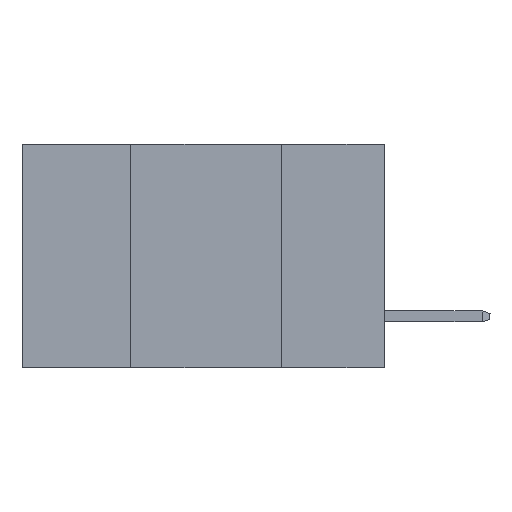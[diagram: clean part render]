
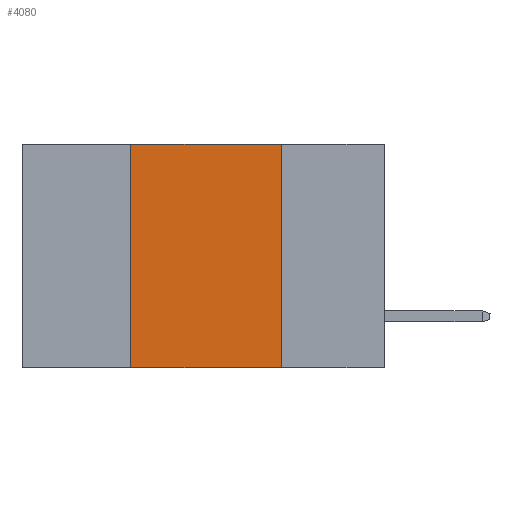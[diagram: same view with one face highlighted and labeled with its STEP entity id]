
A CAD part, left-side view. The second image highlights one B-rep face of the part: STEP entity #4080.
In plain terms, the highlighted planar face has unit normal (-1, 0, 0).
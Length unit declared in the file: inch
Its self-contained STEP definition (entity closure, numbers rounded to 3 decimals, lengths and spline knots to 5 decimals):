
#300 = ORIENTED_EDGE ( 'NONE', *, *, #12971, .F. ) ;
#767 = AXIS2_PLACEMENT_3D ( 'NONE', #18016, #24713, #22697 ) ;
#847 = CARTESIAN_POINT ( 'NONE',  ( 0., 0.42, -0.37 ) ) ;
#1367 = DIRECTION ( 'NONE',  ( 0., -1., 0. ) ) ;
#1958 = VECTOR ( 'NONE', #11075, 39.37008 ) ;
#2663 = EDGE_CURVE ( 'NONE', #6449, #3656, #9830, .T. ) ;
#2944 = LINE ( 'NONE', #5459, #1958 ) ;
#3656 = VERTEX_POINT ( 'NONE', #22191 ) ;
#4080 = ADVANCED_FACE ( 'NONE', ( #14106 ), #7860, .F. ) ;
#5427 = DIRECTION ( 'NONE',  ( 0., 0., -1. ) ) ;
#5459 = CARTESIAN_POINT ( 'NONE',  ( 0., 0.42, -0.37 ) ) ;
#5828 = ORIENTED_EDGE ( 'NONE', *, *, #16334, .F. ) ;
#6449 = VERTEX_POINT ( 'NONE', #847 ) ;
#7342 = LINE ( 'NONE', #15477, #12715 ) ;
#7860 = PLANE ( 'NONE',  #767 ) ;
#8145 = VERTEX_POINT ( 'NONE', #9118 ) ;
#9118 = CARTESIAN_POINT ( 'NONE',  ( 0., 0.42, 0. ) ) ;
#9830 = LINE ( 'NONE', #21991, #11734 ) ;
#11075 = DIRECTION ( 'NONE',  ( 0., 0., 1. ) ) ;
#11734 = VECTOR ( 'NONE', #18245, 39.37008 ) ;
#11840 = VERTEX_POINT ( 'NONE', #18138 ) ;
#12217 = EDGE_CURVE ( 'NONE', #11840, #3656, #15841, .T. ) ;
#12715 = VECTOR ( 'NONE', #1367, 39.37008 ) ;
#12971 = EDGE_CURVE ( 'NONE', #6449, #8145, #2944, .T. ) ;
#13929 = VECTOR ( 'NONE', #5427, 39.37008 ) ;
#14106 = FACE_OUTER_BOUND ( 'NONE', #25862, .T. ) ;
#14360 = ORIENTED_EDGE ( 'NONE', *, *, #12217, .F. ) ;
#15412 = ORIENTED_EDGE ( 'NONE', *, *, #2663, .T. ) ;
#15477 = CARTESIAN_POINT ( 'NONE',  ( 0., 0.6, 0. ) ) ;
#15841 = LINE ( 'NONE', #23746, #13929 ) ;
#16334 = EDGE_CURVE ( 'NONE', #8145, #11840, #7342, .T. ) ;
#18016 = CARTESIAN_POINT ( 'NONE',  ( 0., 0.6, 0. ) ) ;
#18138 = CARTESIAN_POINT ( 'NONE',  ( 0., 0.17, 0. ) ) ;
#18245 = DIRECTION ( 'NONE',  ( 0., -1., 0. ) ) ;
#21991 = CARTESIAN_POINT ( 'NONE',  ( 0., 0.6, -0.37 ) ) ;
#22191 = CARTESIAN_POINT ( 'NONE',  ( 0., 0.17, -0.37 ) ) ;
#22697 = DIRECTION ( 'NONE',  ( 0., 0., -1. ) ) ;
#23746 = CARTESIAN_POINT ( 'NONE',  ( 0., 0.17, -0.37 ) ) ;
#24713 = DIRECTION ( 'NONE',  ( 1., 0., 0. ) ) ;
#25862 = EDGE_LOOP ( 'NONE', ( #14360, #5828, #300, #15412 ) ) ;
